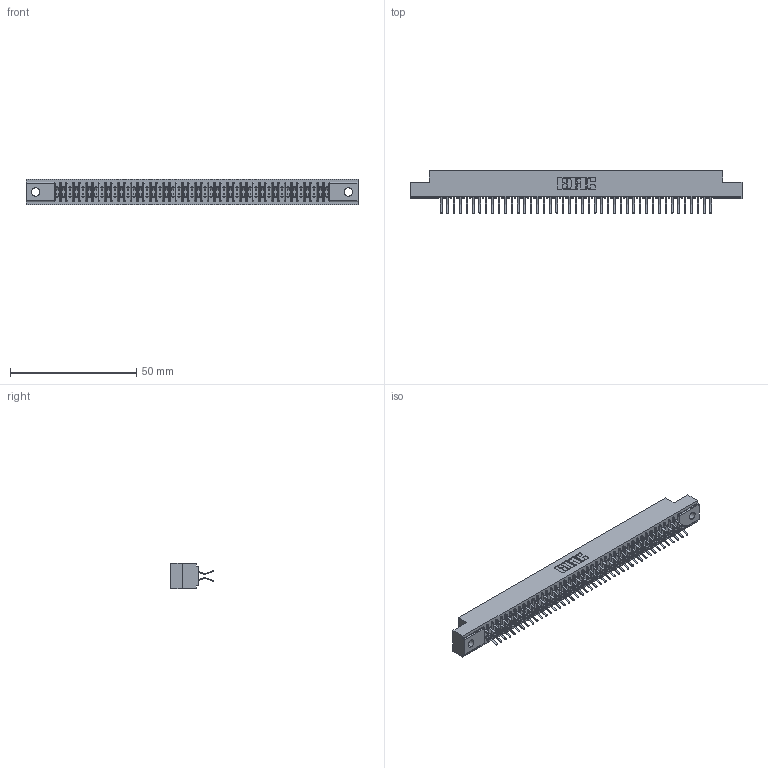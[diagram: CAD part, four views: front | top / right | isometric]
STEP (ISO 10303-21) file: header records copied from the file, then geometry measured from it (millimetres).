
FILE_DESCRIPTION (( 'STEP AP203' ), '1' );
FILE_NAME ('391-086-556-202.STEP', '2018-08-09T16:49:50', ( '' ), ( '' ), 'SwSTEP 2.0', 'SolidWorks 2016', '' );
FILE_SCHEMA (( 'CONFIG_CONTROL_DESIGN' ));
Length unit declared in the file: inch
Products named in the file (3): 341 Part_.128 (3.25) Dia Mounting Holes; 341-292-001_341-292-156; 391-086-556-202
Assembly tree (87 placements, depth 2):
  391-086-556-202
    341 Part_.128 (3.25) Dia Mounting Holes
    341-292-001_341-292-156  x86
Bounding box: 131.44 x 17.07 x 10.16 mm (x, y, z)
Volume: 9694.7 mm3; surface area: 17195.7 mm2
Topology: 87 solids, 87 shells, 6136 faces, 17817 edges, 11558 vertices
Faces by surface type: plane 3508, cylinder 2456, sphere 88, torus 84
Entity records: 52048 total; most frequent: CARTESIAN_POINT 8653, ORIENTED_EDGE 8598, DIRECTION 8401, EDGE_CURVE 4299, VECTOR 3469, LINE 3469, VERTEX_POINT 2718, AXIS2_PLACEMENT_3D 2466
